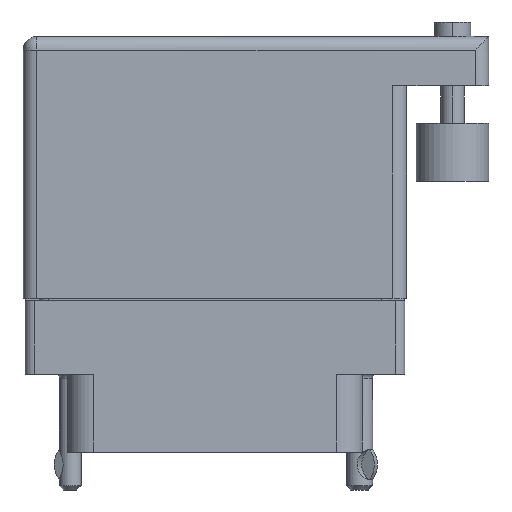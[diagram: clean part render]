
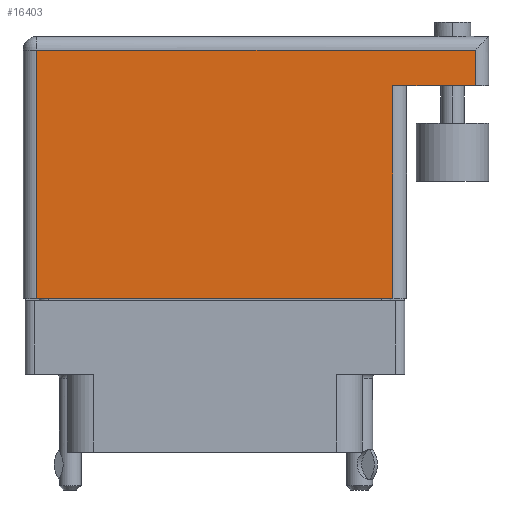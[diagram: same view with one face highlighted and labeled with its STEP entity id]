
A CAD part, front view. The second image highlights one B-rep face of the part: STEP entity #16403.
In plain terms, the highlighted face is planar.
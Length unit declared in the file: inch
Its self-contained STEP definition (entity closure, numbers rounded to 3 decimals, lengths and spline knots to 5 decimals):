
#955 = VECTOR ( 'NONE', #40155, 39.37008 ) ;
#2790 = EDGE_LOOP ( 'NONE', ( #28721, #20978, #7626, #26292, #5732, #14412 ) ) ;
#3102 = EDGE_CURVE ( 'NONE', #32597, #7106, #30622, .T. ) ;
#3724 = CARTESIAN_POINT ( 'NONE',  ( 0.8995, 0.759, 0.3575 ) ) ;
#4616 = EDGE_CURVE ( 'NONE', #22209, #23068, #39157, .T. ) ;
#5046 = CARTESIAN_POINT ( 'NONE',  ( -0.6155, 0.759, 0.3575 ) ) ;
#5154 = CARTESIAN_POINT ( 'NONE',  ( -0.6155, -0.1, 0.3575 ) ) ;
#5288 = EDGE_CURVE ( 'NONE', #35306, #11826, #9025, .T. ) ;
#5732 = ORIENTED_EDGE ( 'NONE', *, *, #5288, .T. ) ;
#6795 = CARTESIAN_POINT ( 'NONE',  ( -0.6155, -0.1, 0.3575 ) ) ;
#6905 = VECTOR ( 'NONE', #20584, 39.37008 ) ;
#7106 = VERTEX_POINT ( 'NONE', #39140 ) ;
#7498 = CARTESIAN_POINT ( 'NONE',  ( -0.6625, 0.806, 0.3575 ) ) ;
#7626 = ORIENTED_EDGE ( 'NONE', *, *, #4616, .F. ) ;
#7762 = DIRECTION ( 'NONE',  ( 0., 1., 0. ) ) ;
#8048 = VECTOR ( 'NONE', #39097, 39.37008 ) ;
#8639 = EDGE_CURVE ( 'NONE', #11826, #32597, #21007, .T. ) ;
#9025 = LINE ( 'NONE', #15506, #27019 ) ;
#11288 = CARTESIAN_POINT ( 'NONE',  ( 0.9465, 0.636, 0.3575 ) ) ;
#11826 = VERTEX_POINT ( 'NONE', #5046 ) ;
#12141 = EDGE_CURVE ( 'NONE', #22209, #35306, #29100, .T. ) ;
#13571 = DIRECTION ( 'NONE',  ( 0., 0., -1. ) ) ;
#14412 = ORIENTED_EDGE ( 'NONE', *, *, #8639, .T. ) ;
#15506 = CARTESIAN_POINT ( 'NONE',  ( -0.6625, 0.759, 0.3575 ) ) ;
#16403 = ADVANCED_FACE ( 'NONE', ( #28827 ), #35546, .F. ) ;
#16589 = VECTOR ( 'NONE', #36116, 39.37008 ) ;
#19420 = CARTESIAN_POINT ( 'NONE',  ( 0.8995, 0.636, 0.3575 ) ) ;
#20541 = VECTOR ( 'NONE', #7762, 39.37008 ) ;
#20584 = DIRECTION ( 'NONE',  ( 0., 1., 0. ) ) ;
#20978 = ORIENTED_EDGE ( 'NONE', *, *, #22916, .T. ) ;
#21007 = LINE ( 'NONE', #5154, #8048 ) ;
#21593 = CARTESIAN_POINT ( 'NONE',  ( 0.6155, 0.636, 0.3575 ) ) ;
#22209 = VERTEX_POINT ( 'NONE', #19420 ) ;
#22916 = EDGE_CURVE ( 'NONE', #7106, #23068, #26082, .T. ) ;
#23068 = VERTEX_POINT ( 'NONE', #21593 ) ;
#25987 = DIRECTION ( 'NONE',  ( -1., 0., 0. ) ) ;
#26082 = LINE ( 'NONE', #29141, #6905 ) ;
#26292 = ORIENTED_EDGE ( 'NONE', *, *, #12141, .T. ) ;
#27019 = VECTOR ( 'NONE', #37463, 39.37008 ) ;
#27562 = CARTESIAN_POINT ( 'NONE',  ( -0.6625, -0.1, 0.3575 ) ) ;
#28721 = ORIENTED_EDGE ( 'NONE', *, *, #3102, .T. ) ;
#28827 = FACE_OUTER_BOUND ( 'NONE', #2790, .T. ) ;
#29100 = LINE ( 'NONE', #29503, #20541 ) ;
#29141 = CARTESIAN_POINT ( 'NONE',  ( 0.6155, 0.636, 0.3575 ) ) ;
#29503 = CARTESIAN_POINT ( 'NONE',  ( 0.8995, 0.806, 0.3575 ) ) ;
#30622 = LINE ( 'NONE', #27562, #955 ) ;
#32597 = VERTEX_POINT ( 'NONE', #6795 ) ;
#35306 = VERTEX_POINT ( 'NONE', #3724 ) ;
#35546 = PLANE ( 'NONE',  #38021 ) ;
#36116 = DIRECTION ( 'NONE',  ( -1., 0., 0. ) ) ;
#37463 = DIRECTION ( 'NONE',  ( -1., 0., 0. ) ) ;
#38021 = AXIS2_PLACEMENT_3D ( 'NONE', #7498, #13571, #25987 ) ;
#39097 = DIRECTION ( 'NONE',  ( 0., -1., 0. ) ) ;
#39140 = CARTESIAN_POINT ( 'NONE',  ( 0.6155, -0.1, 0.3575 ) ) ;
#39157 = LINE ( 'NONE', #11288, #16589 ) ;
#40155 = DIRECTION ( 'NONE',  ( 1., 0., 0. ) ) ;
